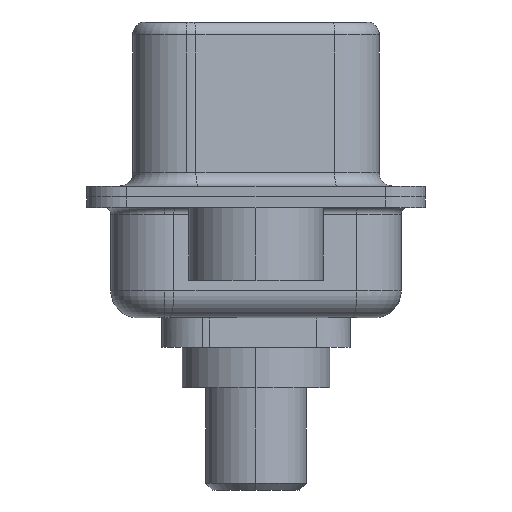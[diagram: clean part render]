
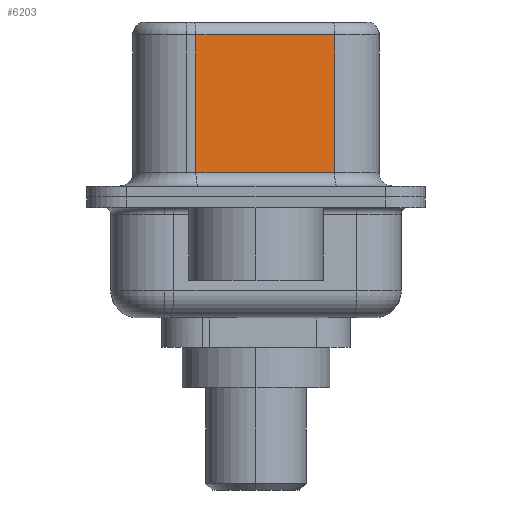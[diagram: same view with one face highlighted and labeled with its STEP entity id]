
A CAD part, left-side view. The second image highlights one B-rep face of the part: STEP entity #6203.
In plain terms, the highlighted planar face has unit normal (-0.985, -0.174, 0).
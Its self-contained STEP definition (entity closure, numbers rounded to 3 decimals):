
#76 = EDGE_CURVE ( 'NONE', #1281, #8403, #12346, .T. ) ;
#483 = FACE_OUTER_BOUND ( 'NONE', #2974, .T. ) ;
#1281 = VERTEX_POINT ( 'NONE', #7316 ) ;
#1384 = CARTESIAN_POINT ( 'NONE',  ( 3.655, 2.233, 0.9 ) ) ;
#2974 = EDGE_LOOP ( 'NONE', ( #4460, #7769, #3659, #6767 ) ) ;
#3364 = VERTEX_POINT ( 'NONE', #7028 ) ;
#3659 = ORIENTED_EDGE ( 'NONE', *, *, #10405, .T. ) ;
#4371 = VECTOR ( 'NONE', #11498, 1000. ) ;
#4460 = ORIENTED_EDGE ( 'NONE', *, *, #76, .F. ) ;
#5514 = DIRECTION ( 'NONE',  ( 0., 0., -1. ) ) ;
#5651 = LINE ( 'NONE', #7336, #8378 ) ;
#5678 = EDGE_CURVE ( 'NONE', #1281, #3364, #8710, .T. ) ;
#5685 = VECTOR ( 'NONE', #9689, 1000. ) ;
#6203 = ADVANCED_FACE ( 'NONE', ( #483 ), #11433, .F. ) ;
#6767 = ORIENTED_EDGE ( 'NONE', *, *, #12518, .T. ) ;
#7028 = CARTESIAN_POINT ( 'NONE',  ( 3.655, 2.233, 6.02 ) ) ;
#7316 = CARTESIAN_POINT ( 'NONE',  ( 4.565, -2.927, 6.02 ) ) ;
#7336 = CARTESIAN_POINT ( 'NONE',  ( 4.565, -2.927, 0.9 ) ) ;
#7479 = CARTESIAN_POINT ( 'NONE',  ( 4.565, -2.927, 6.52 ) ) ;
#7577 = AXIS2_PLACEMENT_3D ( 'NONE', #11295, #11266, #10880 ) ;
#7769 = ORIENTED_EDGE ( 'NONE', *, *, #5678, .T. ) ;
#8378 = VECTOR ( 'NONE', #9328, 1000. ) ;
#8403 = VERTEX_POINT ( 'NONE', #10996 ) ;
#8591 = CARTESIAN_POINT ( 'NONE',  ( 4.565, -2.927, 6.02 ) ) ;
#8710 = LINE ( 'NONE', #8591, #5685 ) ;
#8880 = LINE ( 'NONE', #12497, #11232 ) ;
#9328 = DIRECTION ( 'NONE',  ( 0.174, -0.985, 0. ) ) ;
#9689 = DIRECTION ( 'NONE',  ( -0.174, 0.985, 0. ) ) ;
#10246 = VERTEX_POINT ( 'NONE', #1384 ) ;
#10405 = EDGE_CURVE ( 'NONE', #3364, #10246, #8880, .T. ) ;
#10880 = DIRECTION ( 'NONE',  ( -0.174, 0.985, 0. ) ) ;
#10996 = CARTESIAN_POINT ( 'NONE',  ( 4.565, -2.927, 0.9 ) ) ;
#11232 = VECTOR ( 'NONE', #5514, 1000. ) ;
#11266 = DIRECTION ( 'NONE',  ( 0.985, 0.174, 0. ) ) ;
#11295 = CARTESIAN_POINT ( 'NONE',  ( 4.565, -2.927, 6.52 ) ) ;
#11433 = PLANE ( 'NONE',  #7577 ) ;
#11498 = DIRECTION ( 'NONE',  ( 0., 0., -1. ) ) ;
#12346 = LINE ( 'NONE', #7479, #4371 ) ;
#12497 = CARTESIAN_POINT ( 'NONE',  ( 3.655, 2.233, 6.52 ) ) ;
#12518 = EDGE_CURVE ( 'NONE', #10246, #8403, #5651, .T. ) ;
